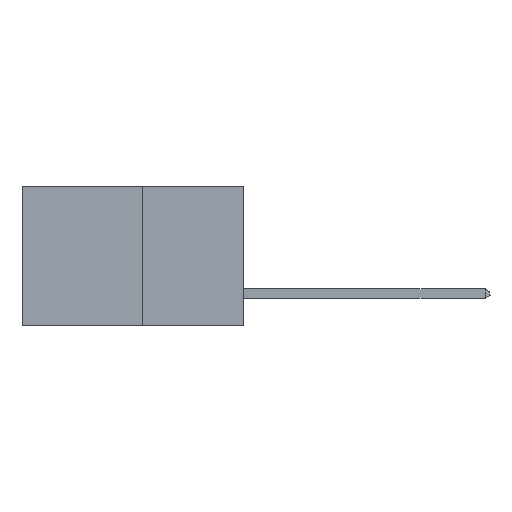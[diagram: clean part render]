
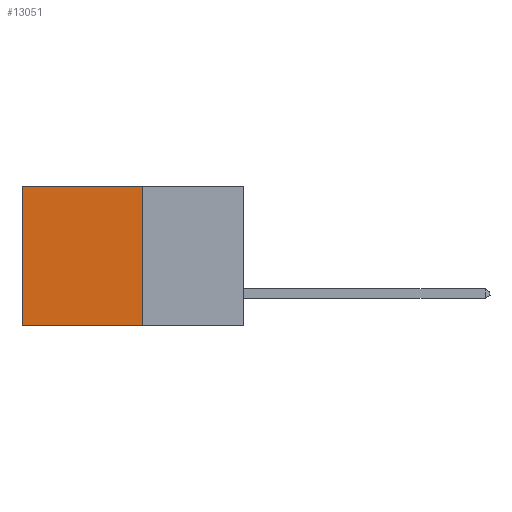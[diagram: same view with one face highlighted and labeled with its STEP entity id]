
A CAD part, left-side view. The second image highlights one B-rep face of the part: STEP entity #13051.
In plain terms, the highlighted planar face has unit normal (-1, 0, 0).
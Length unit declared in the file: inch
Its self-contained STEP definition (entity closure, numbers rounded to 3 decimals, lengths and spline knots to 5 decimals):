
#76 = DIRECTION ( 'NONE',  ( 0., 1., 0. ) ) ;
#463 = LINE ( 'NONE', #5942, #21134 ) ;
#795 = VERTEX_POINT ( 'NONE', #17469 ) ;
#1856 = ORIENTED_EDGE ( 'NONE', *, *, #10752, .T. ) ;
#1913 = PLANE ( 'NONE',  #5638 ) ;
#2217 = LINE ( 'NONE', #12733, #14011 ) ;
#2686 = CARTESIAN_POINT ( 'NONE',  ( 0.277, 0.59, 0. ) ) ;
#2842 = EDGE_CURVE ( 'NONE', #6293, #10232, #463, .T. ) ;
#3596 = DIRECTION ( 'NONE',  ( 1., 0., 0. ) ) ;
#4121 = LINE ( 'NONE', #9712, #9122 ) ;
#4581 = ORIENTED_EDGE ( 'NONE', *, *, #2842, .F. ) ;
#5638 = AXIS2_PLACEMENT_3D ( 'NONE', #13618, #3596, #15311 ) ;
#5838 = EDGE_CURVE ( 'NONE', #795, #6293, #16134, .T. ) ;
#5942 = CARTESIAN_POINT ( 'NONE',  ( 0.277, 0.27, -0.37 ) ) ;
#6293 = VERTEX_POINT ( 'NONE', #11406 ) ;
#6378 = ORIENTED_EDGE ( 'NONE', *, *, #8449, .T. ) ;
#8003 = CARTESIAN_POINT ( 'NONE',  ( 0.277, 0.59, -0.37 ) ) ;
#8449 = EDGE_CURVE ( 'NONE', #13999, #10232, #4121, .T. ) ;
#9122 = VECTOR ( 'NONE', #9689, 39.37008 ) ;
#9372 = CARTESIAN_POINT ( 'NONE',  ( 0.277, 0.27, -0.37 ) ) ;
#9689 = DIRECTION ( 'NONE',  ( 0., 0., -1. ) ) ;
#9712 = CARTESIAN_POINT ( 'NONE',  ( 0.277, 0.59, -0.37 ) ) ;
#10232 = VERTEX_POINT ( 'NONE', #8003 ) ;
#10752 = EDGE_CURVE ( 'NONE', #795, #13999, #2217, .T. ) ;
#11406 = CARTESIAN_POINT ( 'NONE',  ( 0.277, 0.27, -0.37 ) ) ;
#12600 = EDGE_LOOP ( 'NONE', ( #6378, #4581, #14768, #1856 ) ) ;
#12733 = CARTESIAN_POINT ( 'NONE',  ( 0.277, 0.27, 0. ) ) ;
#13051 = ADVANCED_FACE ( 'NONE', ( #15738 ), #1913, .F. ) ;
#13618 = CARTESIAN_POINT ( 'NONE',  ( 0.277, 0.27, -0.37 ) ) ;
#13999 = VERTEX_POINT ( 'NONE', #2686 ) ;
#14011 = VECTOR ( 'NONE', #14400, 39.37008 ) ;
#14400 = DIRECTION ( 'NONE',  ( 0., 1., 0. ) ) ;
#14768 = ORIENTED_EDGE ( 'NONE', *, *, #5838, .F. ) ;
#15311 = DIRECTION ( 'NONE',  ( 0., 0., -1. ) ) ;
#15738 = FACE_OUTER_BOUND ( 'NONE', #12600, .T. ) ;
#16134 = LINE ( 'NONE', #9372, #20463 ) ;
#17176 = DIRECTION ( 'NONE',  ( 0., 0., -1. ) ) ;
#17469 = CARTESIAN_POINT ( 'NONE',  ( 0.277, 0.27, 0. ) ) ;
#20463 = VECTOR ( 'NONE', #17176, 39.37008 ) ;
#21134 = VECTOR ( 'NONE', #76, 39.37008 ) ;
